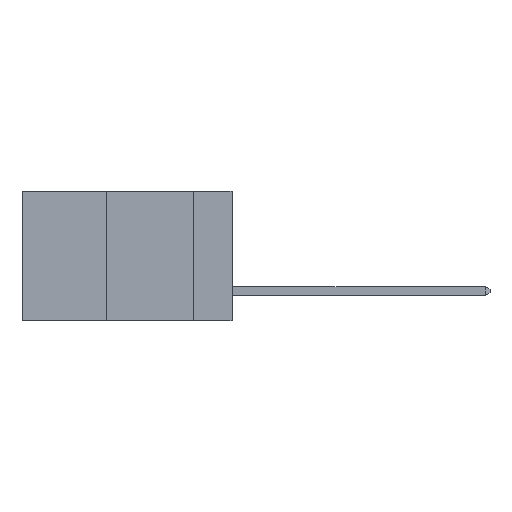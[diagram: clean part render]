
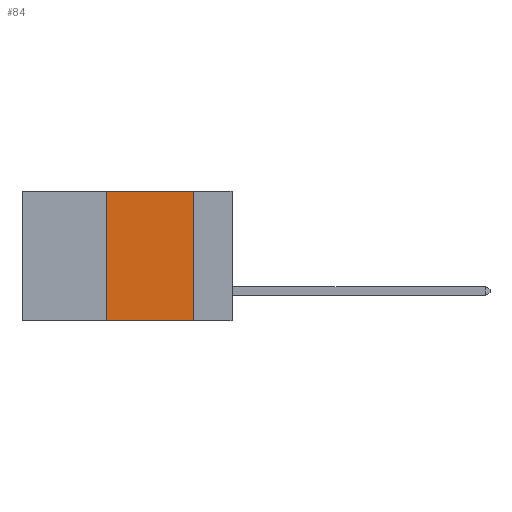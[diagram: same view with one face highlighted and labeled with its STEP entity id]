
A CAD part, left-side view. The second image highlights one B-rep face of the part: STEP entity #84.
In plain terms, the highlighted planar face has unit normal (-1, 0, 0).
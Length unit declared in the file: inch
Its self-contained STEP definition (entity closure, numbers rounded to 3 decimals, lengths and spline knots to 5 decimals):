
#84 = ADVANCED_FACE ( 'NONE', ( #1312 ), #10034, .F. ) ;
#314 = CARTESIAN_POINT ( 'NONE',  ( 0., 0.11, 0. ) ) ;
#542 = EDGE_CURVE ( 'NONE', #15236, #5223, #15609, .T. ) ;
#1297 = VECTOR ( 'NONE', #16081, 39.37008 ) ;
#1312 = FACE_OUTER_BOUND ( 'NONE', #9400, .T. ) ;
#2155 = CARTESIAN_POINT ( 'NONE',  ( 0., 0.36, 0. ) ) ;
#2534 = DIRECTION ( 'NONE',  ( 0., 0., -1. ) ) ;
#2952 = CARTESIAN_POINT ( 'NONE',  ( 0., 0.11, -0.37 ) ) ;
#3557 = DIRECTION ( 'NONE',  ( 0., 0., 1. ) ) ;
#3746 = ORIENTED_EDGE ( 'NONE', *, *, #17363, .F. ) ;
#3762 = ORIENTED_EDGE ( 'NONE', *, *, #542, .F. ) ;
#5223 = VERTEX_POINT ( 'NONE', #314 ) ;
#5470 = ORIENTED_EDGE ( 'NONE', *, *, #17809, .F. ) ;
#5564 = VECTOR ( 'NONE', #2534, 39.37008 ) ;
#5621 = ORIENTED_EDGE ( 'NONE', *, *, #8316, .T. ) ;
#6636 = VECTOR ( 'NONE', #14989, 39.37008 ) ;
#7710 = AXIS2_PLACEMENT_3D ( 'NONE', #16389, #17281, #9116 ) ;
#8031 = CARTESIAN_POINT ( 'NONE',  ( 0., 0.11, 0. ) ) ;
#8067 = CARTESIAN_POINT ( 'NONE',  ( 0., 0.6, -0.37 ) ) ;
#8316 = EDGE_CURVE ( 'NONE', #13142, #14297, #10351, .T. ) ;
#9116 = DIRECTION ( 'NONE',  ( 0., 0., -1. ) ) ;
#9400 = EDGE_LOOP ( 'NONE', ( #3746, #3762, #5470, #5621 ) ) ;
#10034 = PLANE ( 'NONE',  #7710 ) ;
#10351 = LINE ( 'NONE', #8067, #6636 ) ;
#11131 = CARTESIAN_POINT ( 'NONE',  ( 0., 0.36, -0.37 ) ) ;
#12036 = LINE ( 'NONE', #2155, #15336 ) ;
#12961 = LINE ( 'NONE', #8031, #5564 ) ;
#13142 = VERTEX_POINT ( 'NONE', #11131 ) ;
#14297 = VERTEX_POINT ( 'NONE', #2952 ) ;
#14989 = DIRECTION ( 'NONE',  ( 0., -1., 0. ) ) ;
#15236 = VERTEX_POINT ( 'NONE', #16108 ) ;
#15336 = VECTOR ( 'NONE', #3557, 39.37008 ) ;
#15609 = LINE ( 'NONE', #16227, #1297 ) ;
#16081 = DIRECTION ( 'NONE',  ( 0., -1., 0. ) ) ;
#16108 = CARTESIAN_POINT ( 'NONE',  ( 0., 0.36, 0. ) ) ;
#16227 = CARTESIAN_POINT ( 'NONE',  ( 0., 0.6, 0. ) ) ;
#16389 = CARTESIAN_POINT ( 'NONE',  ( 0., 0.6, 0. ) ) ;
#17281 = DIRECTION ( 'NONE',  ( 1., 0., 0. ) ) ;
#17363 = EDGE_CURVE ( 'NONE', #5223, #14297, #12961, .T. ) ;
#17809 = EDGE_CURVE ( 'NONE', #13142, #15236, #12036, .T. ) ;
